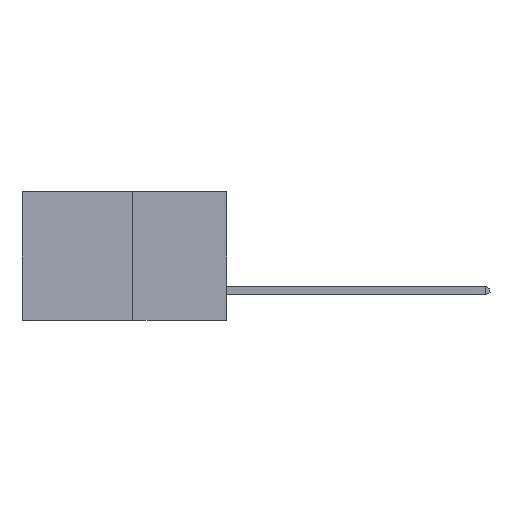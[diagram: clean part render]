
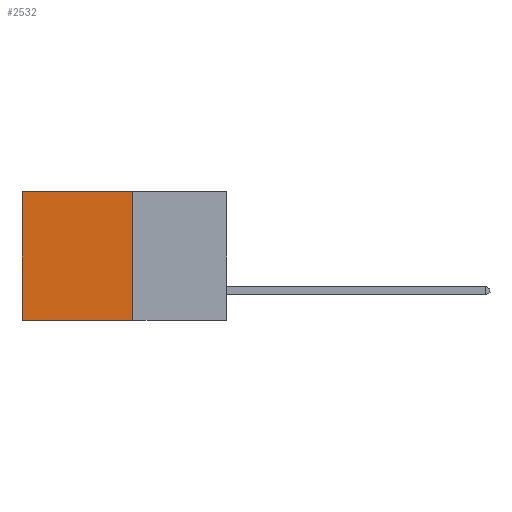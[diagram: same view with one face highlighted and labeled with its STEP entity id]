
A CAD part, left-side view. The second image highlights one B-rep face of the part: STEP entity #2532.
In plain terms, the highlighted planar face has unit normal (-1, 0, 0).
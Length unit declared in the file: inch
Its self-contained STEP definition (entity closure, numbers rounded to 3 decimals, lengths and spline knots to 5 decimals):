
#477 = CARTESIAN_POINT ( 'NONE',  ( 0.277, 0.59, -0.37 ) ) ;
#771 = CARTESIAN_POINT ( 'NONE',  ( 0.277, 0.27, -0.37 ) ) ;
#1283 = EDGE_CURVE ( 'NONE', #5325, #3174, #4577, .T. ) ;
#1382 = CARTESIAN_POINT ( 'NONE',  ( 0.277, 0.27, 0. ) ) ;
#1550 = VECTOR ( 'NONE', #2644, 39.37008 ) ;
#1981 = LINE ( 'NONE', #2425, #1550 ) ;
#2425 = CARTESIAN_POINT ( 'NONE',  ( 0.277, 0.59, -0.37 ) ) ;
#2532 = ADVANCED_FACE ( 'NONE', ( #5293 ), #6410, .F. ) ;
#2644 = DIRECTION ( 'NONE',  ( 0., 0., -1. ) ) ;
#2794 = VECTOR ( 'NONE', #5974, 39.37008 ) ;
#2956 = VERTEX_POINT ( 'NONE', #477 ) ;
#3037 = EDGE_CURVE ( 'NONE', #5325, #7593, #8304, .T. ) ;
#3174 = VERTEX_POINT ( 'NONE', #6997 ) ;
#3350 = VECTOR ( 'NONE', #7765, 39.37008 ) ;
#3762 = ORIENTED_EDGE ( 'NONE', *, *, #1283, .T. ) ;
#4099 = CARTESIAN_POINT ( 'NONE',  ( 0.277, 0.27, -0.37 ) ) ;
#4126 = DIRECTION ( 'NONE',  ( 0., 1., 0. ) ) ;
#4340 = EDGE_CURVE ( 'NONE', #7593, #2956, #7379, .T. ) ;
#4577 = LINE ( 'NONE', #7278, #2794 ) ;
#5293 = FACE_OUTER_BOUND ( 'NONE', #5336, .T. ) ;
#5325 = VERTEX_POINT ( 'NONE', #1382 ) ;
#5336 = EDGE_LOOP ( 'NONE', ( #8253, #5343, #7988, #3762 ) ) ;
#5343 = ORIENTED_EDGE ( 'NONE', *, *, #4340, .F. ) ;
#5560 = VECTOR ( 'NONE', #4126, 39.37008 ) ;
#5974 = DIRECTION ( 'NONE',  ( 0., 1., 0. ) ) ;
#6055 = DIRECTION ( 'NONE',  ( 0., 0., -1. ) ) ;
#6069 = DIRECTION ( 'NONE',  ( 1., 0., 0. ) ) ;
#6111 = CARTESIAN_POINT ( 'NONE',  ( 0.277, 0.27, -0.37 ) ) ;
#6410 = PLANE ( 'NONE',  #7595 ) ;
#6997 = CARTESIAN_POINT ( 'NONE',  ( 0.277, 0.59, 0. ) ) ;
#7278 = CARTESIAN_POINT ( 'NONE',  ( 0.277, 0.27, 0. ) ) ;
#7379 = LINE ( 'NONE', #4099, #5560 ) ;
#7593 = VERTEX_POINT ( 'NONE', #771 ) ;
#7595 = AXIS2_PLACEMENT_3D ( 'NONE', #6111, #6069, #6055 ) ;
#7765 = DIRECTION ( 'NONE',  ( 0., 0., -1. ) ) ;
#7794 = EDGE_CURVE ( 'NONE', #3174, #2956, #1981, .T. ) ;
#7988 = ORIENTED_EDGE ( 'NONE', *, *, #3037, .F. ) ;
#8228 = CARTESIAN_POINT ( 'NONE',  ( 0.277, 0.27, -0.37 ) ) ;
#8253 = ORIENTED_EDGE ( 'NONE', *, *, #7794, .T. ) ;
#8304 = LINE ( 'NONE', #8228, #3350 ) ;
